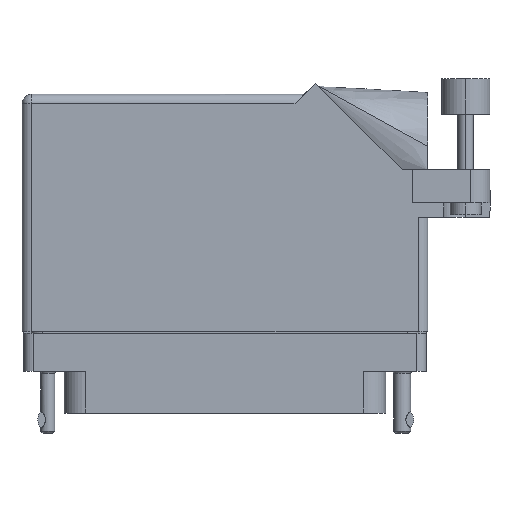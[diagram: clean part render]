
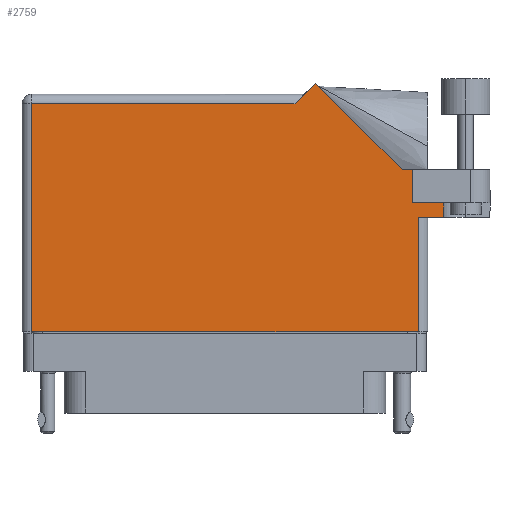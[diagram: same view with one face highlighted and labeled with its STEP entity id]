
A CAD part, front view. The second image highlights one B-rep face of the part: STEP entity #2759.
In plain terms, the highlighted face is planar.
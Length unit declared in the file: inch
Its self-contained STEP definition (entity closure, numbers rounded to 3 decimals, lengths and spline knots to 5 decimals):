
#55 = LINE ( 'NONE', #17253, #23829 ) ;
#393 = LINE ( 'NONE', #54073, #24190 ) ;
#893 = VERTEX_POINT ( 'NONE', #25724 ) ;
#1777 = ORIENTED_EDGE ( 'NONE', *, *, #20349, .T. ) ;
#2223 = DIRECTION ( 'NONE',  ( -1., 0., 0. ) ) ;
#2759 = ADVANCED_FACE ( 'NONE', ( #14434 ), #38867, .F. ) ;
#2841 = VECTOR ( 'NONE', #49691, 39.37008 ) ;
#3603 = CARTESIAN_POINT ( 'NONE',  ( 0.58371, 1.50071, 0.455 ) ) ;
#5963 = CARTESIAN_POINT ( 'NONE',  ( 1.306, 0.637, 0.455 ) ) ;
#6671 = VERTEX_POINT ( 'NONE', #17309 ) ;
#7413 = ORIENTED_EDGE ( 'NONE', *, *, #56380, .T. ) ;
#9249 = ORIENTED_EDGE ( 'NONE', *, *, #15348, .T. ) ;
#9952 = LINE ( 'NONE', #52631, #58873 ) ;
#10044 = VERTEX_POINT ( 'NONE', #57767 ) ;
#10254 = VERTEX_POINT ( 'NONE', #3603 ) ;
#10518 = CARTESIAN_POINT ( 'NONE',  ( 0.513, 1.43, 0.455 ) ) ;
#11053 = VECTOR ( 'NONE', #2223, 39.37008 ) ;
#11524 = VECTOR ( 'NONE', #40744, 39.37008 ) ;
#13102 = EDGE_CURVE ( 'NONE', #51043, #43397, #37042, .T. ) ;
#14027 = EDGE_CURVE ( 'NONE', #57721, #22609, #45053, .T. ) ;
#14434 = FACE_OUTER_BOUND ( 'NONE', #24092, .T. ) ;
#15348 = EDGE_CURVE ( 'NONE', #25592, #10254, #393, .T. ) ;
#15937 = ORIENTED_EDGE ( 'NONE', *, *, #17741, .F. ) ;
#17112 = ORIENTED_EDGE ( 'NONE', *, *, #14027, .T. ) ;
#17253 = CARTESIAN_POINT ( 'NONE',  ( -1.244, -0.1, 0.455 ) ) ;
#17309 = CARTESIAN_POINT ( 'NONE',  ( -1.244, -0.1, 0.455 ) ) ;
#17357 = CARTESIAN_POINT ( 'NONE',  ( 1.206, 0.944, 0.455 ) ) ;
#17493 = VECTOR ( 'NONE', #43994, 39.37008 ) ;
#17679 = VECTOR ( 'NONE', #32716, 39.37008 ) ;
#17741 = EDGE_CURVE ( 'NONE', #57721, #10044, #57308, .T. ) ;
#17870 = CARTESIAN_POINT ( 'NONE',  ( 1.244, -0.1, 0.455 ) ) ;
#18828 = CARTESIAN_POINT ( 'NONE',  ( 1.4075, 1.06177, 0.455 ) ) ;
#18974 = EDGE_CURVE ( 'NONE', #10254, #51043, #56761, .T. ) ;
#20349 = EDGE_CURVE ( 'NONE', #22609, #25592, #9952, .T. ) ;
#21884 = LINE ( 'NONE', #40582, #43446 ) ;
#22042 = EDGE_CURVE ( 'NONE', #893, #39396, #24479, .T. ) ;
#22609 = VERTEX_POINT ( 'NONE', #17357 ) ;
#22996 = CARTESIAN_POINT ( 'NONE',  ( 1.206, 0.731, 0.455 ) ) ;
#23628 = CARTESIAN_POINT ( 'NONE',  ( -1.244, 1.368, 0.455 ) ) ;
#23829 = VECTOR ( 'NONE', #50351, 39.37008 ) ;
#24092 = EDGE_LOOP ( 'NONE', ( #39449, #49495, #50939, #42483, #15937, #17112, #1777, #9249, #24721, #34525, #7413 ) ) ;
#24190 = VECTOR ( 'NONE', #48917, 39.37008 ) ;
#24479 = LINE ( 'NONE', #5963, #28967 ) ;
#24721 = ORIENTED_EDGE ( 'NONE', *, *, #18974, .T. ) ;
#25026 = DIRECTION ( 'NONE',  ( 1., 0., 0. ) ) ;
#25592 = VERTEX_POINT ( 'NONE', #26293 ) ;
#25685 = CARTESIAN_POINT ( 'NONE',  ( 1.4075, 0.637, 0.455 ) ) ;
#25724 = CARTESIAN_POINT ( 'NONE',  ( 1.244, 0.637, 0.455 ) ) ;
#26293 = CARTESIAN_POINT ( 'NONE',  ( 1.14042, 0.944, 0.455 ) ) ;
#28130 = LINE ( 'NONE', #18828, #2841 ) ;
#28967 = VECTOR ( 'NONE', #25026, 39.37008 ) ;
#29130 = DIRECTION ( 'NONE',  ( -1., 0., 0. ) ) ;
#29660 = CARTESIAN_POINT ( 'NONE',  ( -1.306, -0.1, 0.455 ) ) ;
#32716 = DIRECTION ( 'NONE',  ( 0., 1., 0. ) ) ;
#32791 = DIRECTION ( 'NONE',  ( -1., 0., 0. ) ) ;
#34525 = ORIENTED_EDGE ( 'NONE', *, *, #13102, .T. ) ;
#35104 = EDGE_CURVE ( 'NONE', #10044, #39396, #28130, .T. ) ;
#37042 = LINE ( 'NONE', #40414, #11053 ) ;
#37285 = DIRECTION ( 'NONE',  ( 1., 0., 0. ) ) ;
#38867 = PLANE ( 'NONE',  #44835 ) ;
#39053 = CARTESIAN_POINT ( 'NONE',  ( -1.306, 1.43, 0.455 ) ) ;
#39396 = VERTEX_POINT ( 'NONE', #25685 ) ;
#39449 = ORIENTED_EDGE ( 'NONE', *, *, #49727, .T. ) ;
#40414 = CARTESIAN_POINT ( 'NONE',  ( -1.306, 1.368, 0.455 ) ) ;
#40582 = CARTESIAN_POINT ( 'NONE',  ( 1.244, 0.637, 0.455 ) ) ;
#40744 = DIRECTION ( 'NONE',  ( -0.707, -0.707, 0. ) ) ;
#42483 = ORIENTED_EDGE ( 'NONE', *, *, #35104, .F. ) ;
#43397 = VERTEX_POINT ( 'NONE', #23628 ) ;
#43446 = VECTOR ( 'NONE', #59406, 39.37008 ) ;
#43834 = DIRECTION ( 'NONE',  ( 0., 0., -1. ) ) ;
#43994 = DIRECTION ( 'NONE',  ( 1., 0., 0. ) ) ;
#44709 = VECTOR ( 'NONE', #37285, 39.37008 ) ;
#44835 = AXIS2_PLACEMENT_3D ( 'NONE', #39053, #43834, #29130 ) ;
#45053 = LINE ( 'NONE', #22996, #17679 ) ;
#45540 = CARTESIAN_POINT ( 'NONE',  ( 1.206, 0.731, 0.455 ) ) ;
#48431 = EDGE_CURVE ( 'NONE', #51910, #893, #21884, .T. ) ;
#48917 = DIRECTION ( 'NONE',  ( -0.707, 0.707, 0. ) ) ;
#49495 = ORIENTED_EDGE ( 'NONE', *, *, #48431, .T. ) ;
#49691 = DIRECTION ( 'NONE',  ( 0., -1., 0. ) ) ;
#49727 = EDGE_CURVE ( 'NONE', #6671, #51910, #54473, .T. ) ;
#50351 = DIRECTION ( 'NONE',  ( 0., -1., 0. ) ) ;
#50939 = ORIENTED_EDGE ( 'NONE', *, *, #22042, .T. ) ;
#51043 = VERTEX_POINT ( 'NONE', #60346 ) ;
#51910 = VERTEX_POINT ( 'NONE', #17870 ) ;
#52631 = CARTESIAN_POINT ( 'NONE',  ( 1.706, 0.944, 0.455 ) ) ;
#54073 = CARTESIAN_POINT ( 'NONE',  ( 1.14042, 0.944, 0.455 ) ) ;
#54473 = LINE ( 'NONE', #29660, #17493 ) ;
#55510 = CARTESIAN_POINT ( 'NONE',  ( 1.206, 0.731, 0.455 ) ) ;
#56380 = EDGE_CURVE ( 'NONE', #43397, #6671, #55, .T. ) ;
#56761 = LINE ( 'NONE', #10518, #11524 ) ;
#57308 = LINE ( 'NONE', #55510, #44709 ) ;
#57721 = VERTEX_POINT ( 'NONE', #45540 ) ;
#57767 = CARTESIAN_POINT ( 'NONE',  ( 1.4075, 0.731, 0.455 ) ) ;
#58873 = VECTOR ( 'NONE', #32791, 39.37008 ) ;
#59406 = DIRECTION ( 'NONE',  ( 0., 1., 0. ) ) ;
#60346 = CARTESIAN_POINT ( 'NONE',  ( 0.451, 1.368, 0.455 ) ) ;
